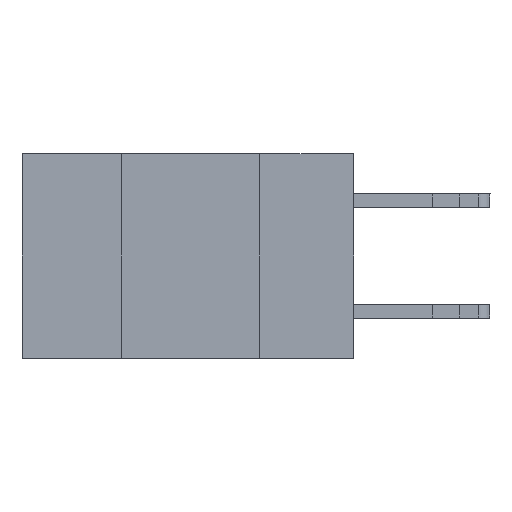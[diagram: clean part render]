
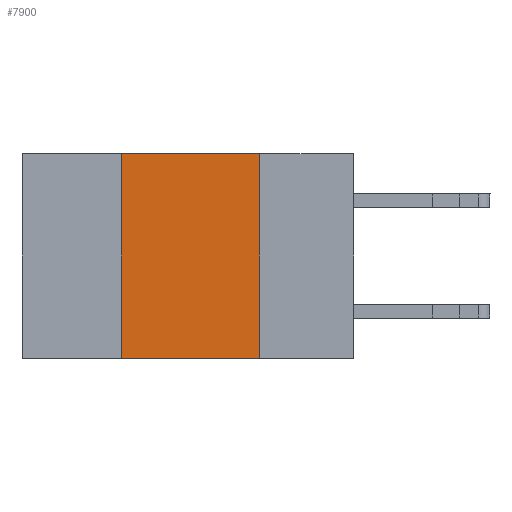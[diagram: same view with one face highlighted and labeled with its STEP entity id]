
A CAD part, left-side view. The second image highlights one B-rep face of the part: STEP entity #7900.
In plain terms, the highlighted planar face has unit normal (-1, 0, 0).
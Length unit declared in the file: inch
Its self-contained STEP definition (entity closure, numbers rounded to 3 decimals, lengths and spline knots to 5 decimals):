
#435 = PLANE ( 'NONE',  #3619 ) ;
#481 = CARTESIAN_POINT ( 'NONE',  ( 0., 0.42, 0. ) ) ;
#898 = CARTESIAN_POINT ( 'NONE',  ( 0., 0.6, 0. ) ) ;
#2736 = ORIENTED_EDGE ( 'NONE', *, *, #23129, .F. ) ;
#2936 = DIRECTION ( 'NONE',  ( 0., 0., -1. ) ) ;
#3203 = EDGE_CURVE ( 'NONE', #21222, #13271, #8842, .T. ) ;
#3386 = CARTESIAN_POINT ( 'NONE',  ( 0., 0.6, -0.37 ) ) ;
#3619 = AXIS2_PLACEMENT_3D ( 'NONE', #898, #11952, #21155 ) ;
#6922 = VECTOR ( 'NONE', #21794, 39.37008 ) ;
#7239 = CARTESIAN_POINT ( 'NONE',  ( 0., 0.42, 0. ) ) ;
#7893 = VECTOR ( 'NONE', #2936, 39.37008 ) ;
#7900 = ADVANCED_FACE ( 'NONE', ( #11691 ), #435, .F. ) ;
#8136 = EDGE_LOOP ( 'NONE', ( #23119, #10196, #2736, #21310 ) ) ;
#8297 = CARTESIAN_POINT ( 'NONE',  ( 0., 0.17, 0. ) ) ;
#8842 = LINE ( 'NONE', #3386, #6922 ) ;
#10196 = ORIENTED_EDGE ( 'NONE', *, *, #14839, .F. ) ;
#10434 = DIRECTION ( 'NONE',  ( 0., -1., 0. ) ) ;
#10552 = CARTESIAN_POINT ( 'NONE',  ( 0., 0.6, 0. ) ) ;
#10566 = LINE ( 'NONE', #19311, #7893 ) ;
#11691 = FACE_OUTER_BOUND ( 'NONE', #8136, .T. ) ;
#11805 = VECTOR ( 'NONE', #15286, 39.37008 ) ;
#11952 = DIRECTION ( 'NONE',  ( 1., 0., 0. ) ) ;
#13271 = VERTEX_POINT ( 'NONE', #20489 ) ;
#14839 = EDGE_CURVE ( 'NONE', #20624, #15172, #21338, .T. ) ;
#15172 = VERTEX_POINT ( 'NONE', #8297 ) ;
#15286 = DIRECTION ( 'NONE',  ( 0., 0., 1. ) ) ;
#18419 = VECTOR ( 'NONE', #10434, 39.37008 ) ;
#19311 = CARTESIAN_POINT ( 'NONE',  ( 0., 0.17, 0. ) ) ;
#19924 = EDGE_CURVE ( 'NONE', #15172, #13271, #10566, .T. ) ;
#20416 = CARTESIAN_POINT ( 'NONE',  ( 0., 0.42, -0.37 ) ) ;
#20489 = CARTESIAN_POINT ( 'NONE',  ( 0., 0.17, -0.37 ) ) ;
#20624 = VERTEX_POINT ( 'NONE', #7239 ) ;
#21155 = DIRECTION ( 'NONE',  ( 0., 0., -1. ) ) ;
#21222 = VERTEX_POINT ( 'NONE', #20416 ) ;
#21310 = ORIENTED_EDGE ( 'NONE', *, *, #3203, .T. ) ;
#21338 = LINE ( 'NONE', #10552, #18419 ) ;
#21794 = DIRECTION ( 'NONE',  ( 0., -1., 0. ) ) ;
#22533 = LINE ( 'NONE', #481, #11805 ) ;
#23119 = ORIENTED_EDGE ( 'NONE', *, *, #19924, .F. ) ;
#23129 = EDGE_CURVE ( 'NONE', #21222, #20624, #22533, .T. ) ;
